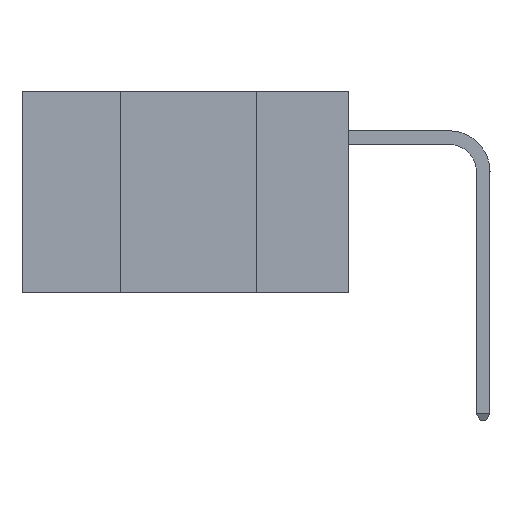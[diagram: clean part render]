
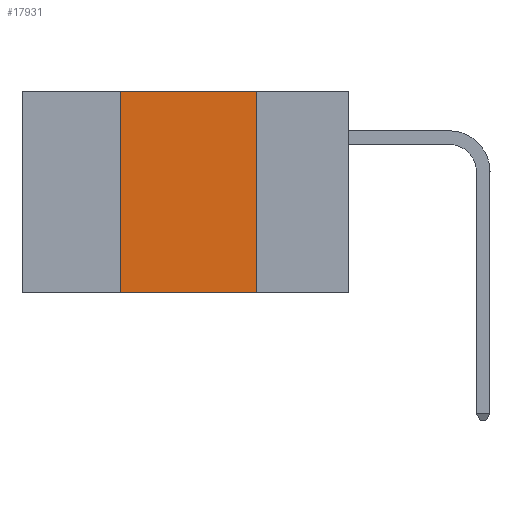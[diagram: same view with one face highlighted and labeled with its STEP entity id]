
A CAD part, left-side view. The second image highlights one B-rep face of the part: STEP entity #17931.
In plain terms, the highlighted planar face has unit normal (-1, 0, 0).
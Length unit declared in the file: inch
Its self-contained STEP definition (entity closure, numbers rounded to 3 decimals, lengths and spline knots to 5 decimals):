
#2386 = FACE_OUTER_BOUND ( 'NONE', #33605, .T. ) ;
#2949 = ORIENTED_EDGE ( 'NONE', *, *, #25485, .T. ) ;
#3640 = LINE ( 'NONE', #47212, #5939 ) ;
#5463 = EDGE_CURVE ( 'NONE', #35257, #45863, #45718, .T. ) ;
#5939 = VECTOR ( 'NONE', #14483, 39.37008 ) ;
#6195 = DIRECTION ( 'NONE',  ( 1., 0., 0. ) ) ;
#8660 = CARTESIAN_POINT ( 'NONE',  ( 0., 0.17, 0. ) ) ;
#8749 = VECTOR ( 'NONE', #38481, 39.37008 ) ;
#8832 = VECTOR ( 'NONE', #18316, 39.37008 ) ;
#8958 = ORIENTED_EDGE ( 'NONE', *, *, #16101, .F. ) ;
#9785 = VECTOR ( 'NONE', #45111, 39.37008 ) ;
#14319 = CARTESIAN_POINT ( 'NONE',  ( 0., 0.17, -0.37 ) ) ;
#14373 = CARTESIAN_POINT ( 'NONE',  ( 0., 0.42, 0. ) ) ;
#14483 = DIRECTION ( 'NONE',  ( 0., -1., 0. ) ) ;
#15181 = VERTEX_POINT ( 'NONE', #45552 ) ;
#16101 = EDGE_CURVE ( 'NONE', #28285, #35257, #3640, .T. ) ;
#17931 = ADVANCED_FACE ( 'NONE', ( #2386 ), #34957, .F. ) ;
#18316 = DIRECTION ( 'NONE',  ( 0., 0., 1. ) ) ;
#18810 = CARTESIAN_POINT ( 'NONE',  ( 0., 0.6, 0. ) ) ;
#20770 = LINE ( 'NONE', #39596, #8832 ) ;
#24070 = EDGE_CURVE ( 'NONE', #15181, #28285, #20770, .T. ) ;
#25485 = EDGE_CURVE ( 'NONE', #15181, #45863, #36586, .T. ) ;
#28285 = VERTEX_POINT ( 'NONE', #14373 ) ;
#30091 = CARTESIAN_POINT ( 'NONE',  ( 0., 0.17, 0. ) ) ;
#30445 = AXIS2_PLACEMENT_3D ( 'NONE', #18810, #6195, #35758 ) ;
#32247 = ORIENTED_EDGE ( 'NONE', *, *, #24070, .F. ) ;
#33605 = EDGE_LOOP ( 'NONE', ( #41535, #8958, #32247, #2949 ) ) ;
#34957 = PLANE ( 'NONE',  #30445 ) ;
#35257 = VERTEX_POINT ( 'NONE', #8660 ) ;
#35758 = DIRECTION ( 'NONE',  ( 0., 0., -1. ) ) ;
#36586 = LINE ( 'NONE', #41237, #8749 ) ;
#38481 = DIRECTION ( 'NONE',  ( 0., -1., 0. ) ) ;
#39596 = CARTESIAN_POINT ( 'NONE',  ( 0., 0.42, 0. ) ) ;
#41237 = CARTESIAN_POINT ( 'NONE',  ( 0., 0.6, -0.37 ) ) ;
#41535 = ORIENTED_EDGE ( 'NONE', *, *, #5463, .F. ) ;
#45111 = DIRECTION ( 'NONE',  ( 0., 0., -1. ) ) ;
#45552 = CARTESIAN_POINT ( 'NONE',  ( 0., 0.42, -0.37 ) ) ;
#45718 = LINE ( 'NONE', #30091, #9785 ) ;
#45863 = VERTEX_POINT ( 'NONE', #14319 ) ;
#47212 = CARTESIAN_POINT ( 'NONE',  ( 0., 0.6, 0. ) ) ;
